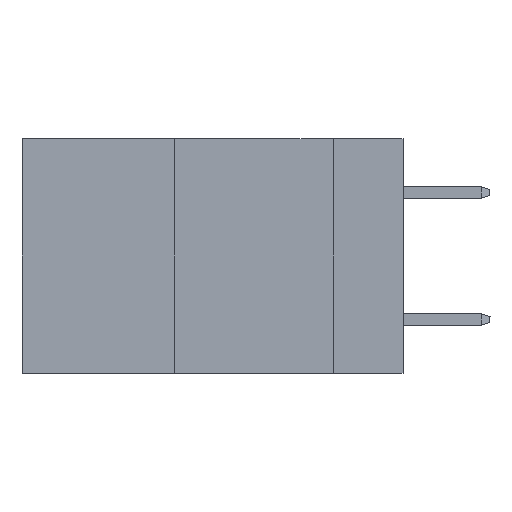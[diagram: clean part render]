
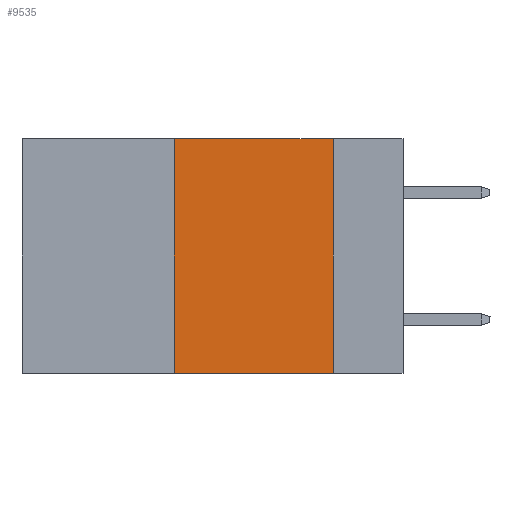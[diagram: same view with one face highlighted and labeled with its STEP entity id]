
A CAD part, left-side view. The second image highlights one B-rep face of the part: STEP entity #9535.
In plain terms, the highlighted planar face has unit normal (-1, 0, 0).
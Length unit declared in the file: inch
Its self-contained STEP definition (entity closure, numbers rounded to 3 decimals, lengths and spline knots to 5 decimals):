
#443 = LINE ( 'NONE', #23009, #23238 ) ;
#786 = VERTEX_POINT ( 'NONE', #9731 ) ;
#2157 = ORIENTED_EDGE ( 'NONE', *, *, #7414, .F. ) ;
#3637 = VERTEX_POINT ( 'NONE', #21208 ) ;
#4004 = EDGE_CURVE ( 'NONE', #10519, #3637, #4957, .T. ) ;
#4957 = LINE ( 'NONE', #22781, #16008 ) ;
#5196 = CARTESIAN_POINT ( 'NONE',  ( 0., 0.6, -0.37 ) ) ;
#6535 = CARTESIAN_POINT ( 'NONE',  ( 0., 0.6, 0. ) ) ;
#7414 = EDGE_CURVE ( 'NONE', #14947, #10519, #20243, .T. ) ;
#8505 = VECTOR ( 'NONE', #27595, 39.37008 ) ;
#9535 = ADVANCED_FACE ( 'NONE', ( #21653 ), #28132, .F. ) ;
#9731 = CARTESIAN_POINT ( 'NONE',  ( 0., 0.36, -0.37 ) ) ;
#9868 = ORIENTED_EDGE ( 'NONE', *, *, #4004, .F. ) ;
#10360 = CARTESIAN_POINT ( 'NONE',  ( 0., 0.6, 0. ) ) ;
#10519 = VERTEX_POINT ( 'NONE', #18041 ) ;
#11291 = CARTESIAN_POINT ( 'NONE',  ( 0., 0.36, 0. ) ) ;
#12653 = EDGE_LOOP ( 'NONE', ( #9868, #2157, #18924, #25468 ) ) ;
#13326 = EDGE_CURVE ( 'NONE', #786, #14947, #443, .T. ) ;
#14598 = VECTOR ( 'NONE', #24512, 39.37008 ) ;
#14947 = VERTEX_POINT ( 'NONE', #11291 ) ;
#16008 = VECTOR ( 'NONE', #27074, 39.37008 ) ;
#16230 = DIRECTION ( 'NONE',  ( 0., 0., 1. ) ) ;
#17515 = AXIS2_PLACEMENT_3D ( 'NONE', #10360, #23276, #25499 ) ;
#18041 = CARTESIAN_POINT ( 'NONE',  ( 0., 0.11, 0. ) ) ;
#18924 = ORIENTED_EDGE ( 'NONE', *, *, #13326, .F. ) ;
#19203 = LINE ( 'NONE', #5196, #8505 ) ;
#20243 = LINE ( 'NONE', #6535, #14598 ) ;
#21208 = CARTESIAN_POINT ( 'NONE',  ( 0., 0.11, -0.37 ) ) ;
#21653 = FACE_OUTER_BOUND ( 'NONE', #12653, .T. ) ;
#22781 = CARTESIAN_POINT ( 'NONE',  ( 0., 0.11, 0. ) ) ;
#23009 = CARTESIAN_POINT ( 'NONE',  ( 0., 0.36, 0. ) ) ;
#23238 = VECTOR ( 'NONE', #16230, 39.37008 ) ;
#23276 = DIRECTION ( 'NONE',  ( 1., 0., 0. ) ) ;
#24512 = DIRECTION ( 'NONE',  ( 0., -1., 0. ) ) ;
#25468 = ORIENTED_EDGE ( 'NONE', *, *, #26206, .T. ) ;
#25499 = DIRECTION ( 'NONE',  ( 0., 0., -1. ) ) ;
#26206 = EDGE_CURVE ( 'NONE', #786, #3637, #19203, .T. ) ;
#27074 = DIRECTION ( 'NONE',  ( 0., 0., -1. ) ) ;
#27595 = DIRECTION ( 'NONE',  ( 0., -1., 0. ) ) ;
#28132 = PLANE ( 'NONE',  #17515 ) ;
